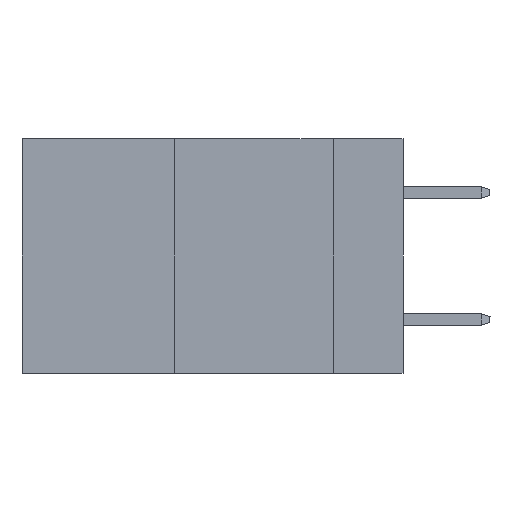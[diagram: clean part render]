
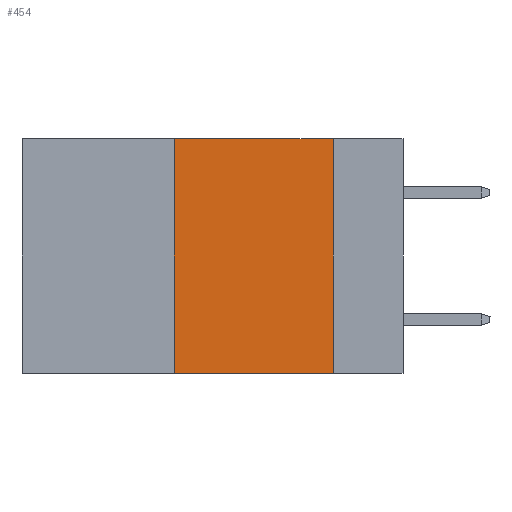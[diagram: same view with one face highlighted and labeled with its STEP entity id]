
A CAD part, left-side view. The second image highlights one B-rep face of the part: STEP entity #454.
In plain terms, the highlighted planar face has unit normal (-1, 0, 0).
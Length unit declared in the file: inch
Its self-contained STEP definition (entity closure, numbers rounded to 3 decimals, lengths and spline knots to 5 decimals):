
#454 = ADVANCED_FACE ( 'NONE', ( #2193 ), #19439, .F. ) ;
#702 = CARTESIAN_POINT ( 'NONE',  ( 0., 0.11, 0. ) ) ;
#945 = LINE ( 'NONE', #32099, #1117 ) ;
#1117 = VECTOR ( 'NONE', #9004, 39.37008 ) ;
#1828 = DIRECTION ( 'NONE',  ( 0., 0., -1. ) ) ;
#1875 = VECTOR ( 'NONE', #8828, 39.37008 ) ;
#2193 = FACE_OUTER_BOUND ( 'NONE', #12402, .T. ) ;
#3229 = CARTESIAN_POINT ( 'NONE',  ( 0., 0.11, 0. ) ) ;
#3864 = EDGE_CURVE ( 'NONE', #29106, #36711, #6395, .T. ) ;
#5368 = CARTESIAN_POINT ( 'NONE',  ( 0., 0.6, 0. ) ) ;
#6395 = LINE ( 'NONE', #3229, #1875 ) ;
#7764 = CARTESIAN_POINT ( 'NONE',  ( 0., 0.36, -0.37 ) ) ;
#8245 = EDGE_CURVE ( 'NONE', #10440, #29106, #945, .T. ) ;
#8797 = CARTESIAN_POINT ( 'NONE',  ( 0., 0.36, 0. ) ) ;
#8828 = DIRECTION ( 'NONE',  ( 0., 0., -1. ) ) ;
#9004 = DIRECTION ( 'NONE',  ( 0., -1., 0. ) ) ;
#10440 = VERTEX_POINT ( 'NONE', #19381 ) ;
#10895 = CARTESIAN_POINT ( 'NONE',  ( 0., 0.6, -0.37 ) ) ;
#12402 = EDGE_LOOP ( 'NONE', ( #14491, #20098, #33722, #15040 ) ) ;
#14491 = ORIENTED_EDGE ( 'NONE', *, *, #3864, .F. ) ;
#15040 = ORIENTED_EDGE ( 'NONE', *, *, #25563, .T. ) ;
#17618 = AXIS2_PLACEMENT_3D ( 'NONE', #5368, #28079, #1828 ) ;
#19381 = CARTESIAN_POINT ( 'NONE',  ( 0., 0.36, 0. ) ) ;
#19439 = PLANE ( 'NONE',  #17618 ) ;
#20098 = ORIENTED_EDGE ( 'NONE', *, *, #8245, .F. ) ;
#20273 = DIRECTION ( 'NONE',  ( 0., 0., 1. ) ) ;
#22708 = LINE ( 'NONE', #8797, #26814 ) ;
#24361 = EDGE_CURVE ( 'NONE', #29404, #10440, #22708, .T. ) ;
#25175 = LINE ( 'NONE', #10895, #30376 ) ;
#25563 = EDGE_CURVE ( 'NONE', #29404, #36711, #25175, .T. ) ;
#26814 = VECTOR ( 'NONE', #20273, 39.37008 ) ;
#27974 = DIRECTION ( 'NONE',  ( 0., -1., 0. ) ) ;
#28079 = DIRECTION ( 'NONE',  ( 1., 0., 0. ) ) ;
#28526 = CARTESIAN_POINT ( 'NONE',  ( 0., 0.11, -0.37 ) ) ;
#29106 = VERTEX_POINT ( 'NONE', #702 ) ;
#29404 = VERTEX_POINT ( 'NONE', #7764 ) ;
#30376 = VECTOR ( 'NONE', #27974, 39.37008 ) ;
#32099 = CARTESIAN_POINT ( 'NONE',  ( 0., 0.6, 0. ) ) ;
#33722 = ORIENTED_EDGE ( 'NONE', *, *, #24361, .F. ) ;
#36711 = VERTEX_POINT ( 'NONE', #28526 ) ;
